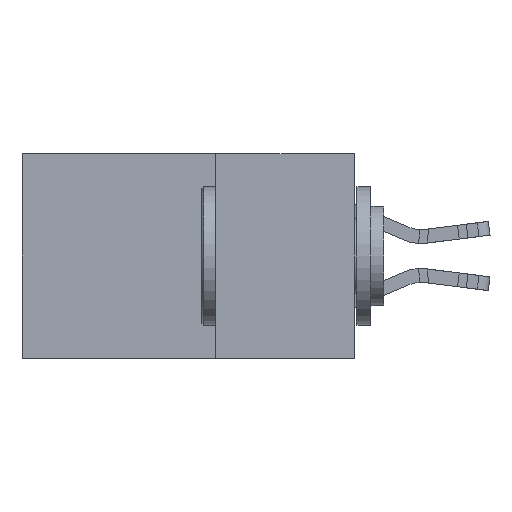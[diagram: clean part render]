
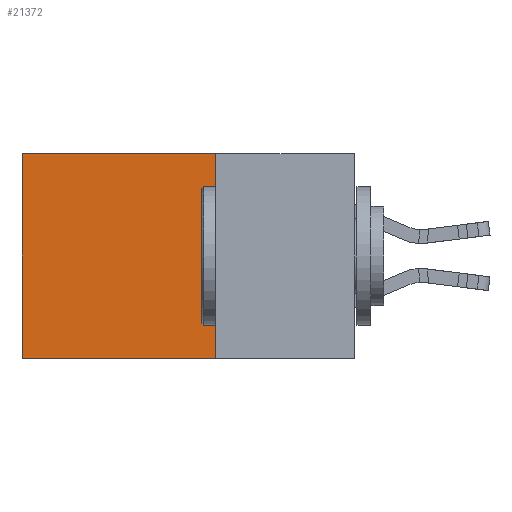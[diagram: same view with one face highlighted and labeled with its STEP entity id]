
A CAD part, left-side view. The second image highlights one B-rep face of the part: STEP entity #21372.
In plain terms, the highlighted planar face has unit normal (-1, 0, 0).
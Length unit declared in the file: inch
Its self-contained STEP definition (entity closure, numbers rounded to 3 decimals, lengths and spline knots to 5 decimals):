
#65 = LINE ( 'NONE', #33751, #12636 ) ;
#1957 = CARTESIAN_POINT ( 'NONE',  ( 0.298, 0.25, -0.37 ) ) ;
#2740 = LINE ( 'NONE', #29697, #9019 ) ;
#3508 = VERTEX_POINT ( 'NONE', #30713 ) ;
#4282 = CARTESIAN_POINT ( 'NONE',  ( 0.298, 0.6, 0. ) ) ;
#5206 = CARTESIAN_POINT ( 'NONE',  ( 0.298, 0.25, 0. ) ) ;
#5651 = ORIENTED_EDGE ( 'NONE', *, *, #11742, .F. ) ;
#6197 = EDGE_CURVE ( 'NONE', #3508, #19429, #15828, .T. ) ;
#7909 = PLANE ( 'NONE',  #9251 ) ;
#8355 = VERTEX_POINT ( 'NONE', #23679 ) ;
#9019 = VECTOR ( 'NONE', #11358, 39.37008 ) ;
#9251 = AXIS2_PLACEMENT_3D ( 'NONE', #5206, #10580, #28922 ) ;
#10216 = FACE_OUTER_BOUND ( 'NONE', #22751, .T. ) ;
#10580 = DIRECTION ( 'NONE',  ( 1., 0., 0. ) ) ;
#11358 = DIRECTION ( 'NONE',  ( 0., 1., 0. ) ) ;
#11605 = EDGE_CURVE ( 'NONE', #19429, #8355, #26179, .T. ) ;
#11742 = EDGE_CURVE ( 'NONE', #3508, #32146, #65, .T. ) ;
#12344 = DIRECTION ( 'NONE',  ( 0., 1., 0. ) ) ;
#12636 = VECTOR ( 'NONE', #15423, 39.37008 ) ;
#14272 = ORIENTED_EDGE ( 'NONE', *, *, #11605, .T. ) ;
#15423 = DIRECTION ( 'NONE',  ( 0., 0., -1. ) ) ;
#15828 = LINE ( 'NONE', #20275, #28942 ) ;
#17810 = ORIENTED_EDGE ( 'NONE', *, *, #6197, .T. ) ;
#19429 = VERTEX_POINT ( 'NONE', #24868 ) ;
#20275 = CARTESIAN_POINT ( 'NONE',  ( 0.298, 0.25, 0. ) ) ;
#21372 = ADVANCED_FACE ( 'NONE', ( #10216 ), #7909, .F. ) ;
#22751 = EDGE_LOOP ( 'NONE', ( #14272, #23823, #5651, #17810 ) ) ;
#23679 = CARTESIAN_POINT ( 'NONE',  ( 0.298, 0.6, -0.37 ) ) ;
#23715 = VECTOR ( 'NONE', #28029, 39.37008 ) ;
#23823 = ORIENTED_EDGE ( 'NONE', *, *, #28539, .F. ) ;
#24868 = CARTESIAN_POINT ( 'NONE',  ( 0.298, 0.6, 0. ) ) ;
#26179 = LINE ( 'NONE', #4282, #23715 ) ;
#28029 = DIRECTION ( 'NONE',  ( 0., 0., -1. ) ) ;
#28539 = EDGE_CURVE ( 'NONE', #32146, #8355, #2740, .T. ) ;
#28922 = DIRECTION ( 'NONE',  ( 0., 0., -1. ) ) ;
#28942 = VECTOR ( 'NONE', #12344, 39.37008 ) ;
#29697 = CARTESIAN_POINT ( 'NONE',  ( 0.298, 0.25, -0.37 ) ) ;
#30713 = CARTESIAN_POINT ( 'NONE',  ( 0.298, 0.25, 0. ) ) ;
#32146 = VERTEX_POINT ( 'NONE', #1957 ) ;
#33751 = CARTESIAN_POINT ( 'NONE',  ( 0.298, 0.25, 0. ) ) ;
